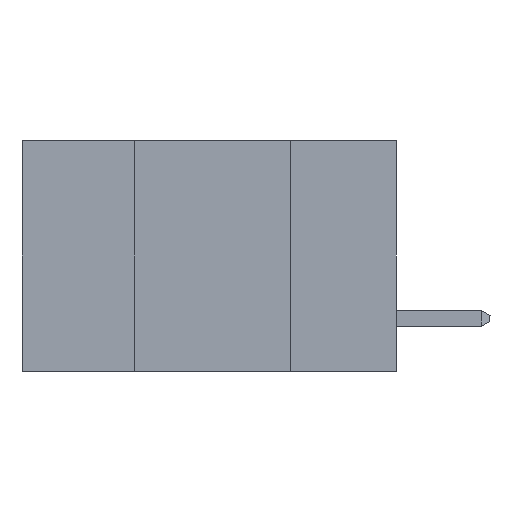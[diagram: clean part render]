
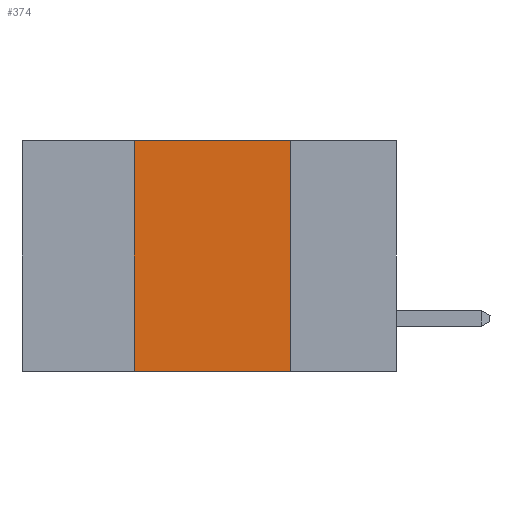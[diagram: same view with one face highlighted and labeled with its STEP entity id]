
A CAD part, left-side view. The second image highlights one B-rep face of the part: STEP entity #374.
In plain terms, the highlighted planar face has unit normal (-1, 0, 0).
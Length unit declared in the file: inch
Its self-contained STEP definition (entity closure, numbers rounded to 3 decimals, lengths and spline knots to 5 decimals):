
#231 = CARTESIAN_POINT ( 'NONE',  ( 0., 0.6, -0.37 ) ) ;
#374 = ADVANCED_FACE ( 'NONE', ( #9579 ), #3988, .F. ) ;
#611 = CARTESIAN_POINT ( 'NONE',  ( 0., 0.6, 0. ) ) ;
#1570 = LINE ( 'NONE', #4543, #7857 ) ;
#1718 = VERTEX_POINT ( 'NONE', #2764 ) ;
#1752 = ORIENTED_EDGE ( 'NONE', *, *, #3027, .F. ) ;
#1967 = EDGE_LOOP ( 'NONE', ( #1752, #6776, #6085, #9437 ) ) ;
#2764 = CARTESIAN_POINT ( 'NONE',  ( 0., 0.42, 0. ) ) ;
#2782 = VECTOR ( 'NONE', #3408, 39.37008 ) ;
#3013 = DIRECTION ( 'NONE',  ( 0., 0., -1. ) ) ;
#3027 = EDGE_CURVE ( 'NONE', #9831, #8519, #5881, .T. ) ;
#3087 = CARTESIAN_POINT ( 'NONE',  ( 0., 0.42, 0. ) ) ;
#3196 = LINE ( 'NONE', #3087, #4531 ) ;
#3408 = DIRECTION ( 'NONE',  ( 0., 0., -1. ) ) ;
#3874 = DIRECTION ( 'NONE',  ( 0., -1., 0. ) ) ;
#3952 = DIRECTION ( 'NONE',  ( 1., 0., 0. ) ) ;
#3988 = PLANE ( 'NONE',  #6943 ) ;
#4531 = VECTOR ( 'NONE', #9140, 39.37008 ) ;
#4543 = CARTESIAN_POINT ( 'NONE',  ( 0., 0.6, 0. ) ) ;
#5811 = CARTESIAN_POINT ( 'NONE',  ( 0., 0.17, -0.37 ) ) ;
#5881 = LINE ( 'NONE', #6109, #2782 ) ;
#6085 = ORIENTED_EDGE ( 'NONE', *, *, #9397, .F. ) ;
#6109 = CARTESIAN_POINT ( 'NONE',  ( 0., 0.17, 0. ) ) ;
#6514 = CARTESIAN_POINT ( 'NONE',  ( 0., 0.17, 0. ) ) ;
#6776 = ORIENTED_EDGE ( 'NONE', *, *, #9772, .F. ) ;
#6800 = VECTOR ( 'NONE', #3874, 39.37008 ) ;
#6943 = AXIS2_PLACEMENT_3D ( 'NONE', #611, #3952, #3013 ) ;
#7327 = LINE ( 'NONE', #231, #6800 ) ;
#7819 = CARTESIAN_POINT ( 'NONE',  ( 0., 0.42, -0.37 ) ) ;
#7857 = VECTOR ( 'NONE', #10602, 39.37008 ) ;
#8519 = VERTEX_POINT ( 'NONE', #5811 ) ;
#9140 = DIRECTION ( 'NONE',  ( 0., 0., 1. ) ) ;
#9397 = EDGE_CURVE ( 'NONE', #9686, #1718, #3196, .T. ) ;
#9437 = ORIENTED_EDGE ( 'NONE', *, *, #10244, .T. ) ;
#9579 = FACE_OUTER_BOUND ( 'NONE', #1967, .T. ) ;
#9686 = VERTEX_POINT ( 'NONE', #7819 ) ;
#9772 = EDGE_CURVE ( 'NONE', #1718, #9831, #1570, .T. ) ;
#9831 = VERTEX_POINT ( 'NONE', #6514 ) ;
#10244 = EDGE_CURVE ( 'NONE', #9686, #8519, #7327, .T. ) ;
#10602 = DIRECTION ( 'NONE',  ( 0., -1., 0. ) ) ;
